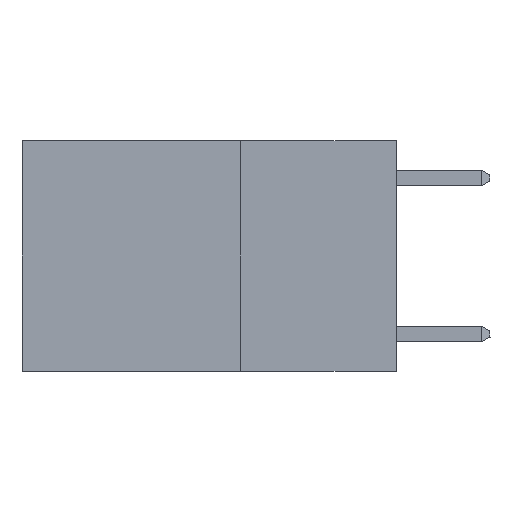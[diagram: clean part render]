
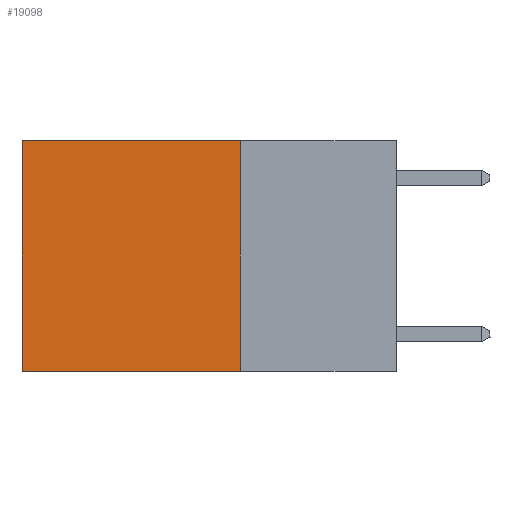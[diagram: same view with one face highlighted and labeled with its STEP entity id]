
A CAD part, left-side view. The second image highlights one B-rep face of the part: STEP entity #19098.
In plain terms, the highlighted planar face has unit normal (-1, 0, 0).
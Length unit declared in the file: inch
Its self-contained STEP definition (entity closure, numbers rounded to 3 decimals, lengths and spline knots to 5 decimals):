
#115 = CARTESIAN_POINT ( 'NONE',  ( 0.2625, 0.25, -0.37 ) ) ;
#633 = VECTOR ( 'NONE', #17100, 39.37008 ) ;
#937 = LINE ( 'NONE', #3452, #633 ) ;
#1127 = VERTEX_POINT ( 'NONE', #10724 ) ;
#1497 = EDGE_CURVE ( 'NONE', #13626, #9747, #11263, .T. ) ;
#1916 = DIRECTION ( 'NONE',  ( 0., 1., 0. ) ) ;
#2401 = PLANE ( 'NONE',  #7208 ) ;
#3452 = CARTESIAN_POINT ( 'NONE',  ( 0.2625, 0.25, 0. ) ) ;
#3915 = VECTOR ( 'NONE', #16270, 39.37008 ) ;
#4305 = ORIENTED_EDGE ( 'NONE', *, *, #17801, .F. ) ;
#5739 = ORIENTED_EDGE ( 'NONE', *, *, #16475, .T. ) ;
#6186 = DIRECTION ( 'NONE',  ( 0., 0., -1. ) ) ;
#6295 = CARTESIAN_POINT ( 'NONE',  ( 0.2625, 0.6, 0. ) ) ;
#7208 = AXIS2_PLACEMENT_3D ( 'NONE', #19495, #9434, #21037 ) ;
#7771 = CARTESIAN_POINT ( 'NONE',  ( 0.2625, 0.25, 0. ) ) ;
#8571 = LINE ( 'NONE', #7771, #3915 ) ;
#8834 = CARTESIAN_POINT ( 'NONE',  ( 0.2625, 0.6, -0.37 ) ) ;
#8914 = ORIENTED_EDGE ( 'NONE', *, *, #14545, .F. ) ;
#9434 = DIRECTION ( 'NONE',  ( 1., 0., 0. ) ) ;
#9747 = VERTEX_POINT ( 'NONE', #8834 ) ;
#10724 = CARTESIAN_POINT ( 'NONE',  ( 0.2625, 0.25, 0. ) ) ;
#10732 = VECTOR ( 'NONE', #6186, 39.37008 ) ;
#11263 = LINE ( 'NONE', #6295, #10732 ) ;
#12610 = ORIENTED_EDGE ( 'NONE', *, *, #1497, .T. ) ;
#13084 = FACE_OUTER_BOUND ( 'NONE', #19761, .T. ) ;
#13626 = VERTEX_POINT ( 'NONE', #19842 ) ;
#14545 = EDGE_CURVE ( 'NONE', #17948, #9747, #17337, .T. ) ;
#16270 = DIRECTION ( 'NONE',  ( 0., 0., -1. ) ) ;
#16475 = EDGE_CURVE ( 'NONE', #1127, #13626, #937, .T. ) ;
#17100 = DIRECTION ( 'NONE',  ( 0., 1., 0. ) ) ;
#17337 = LINE ( 'NONE', #115, #17551 ) ;
#17551 = VECTOR ( 'NONE', #1916, 39.37008 ) ;
#17801 = EDGE_CURVE ( 'NONE', #1127, #17948, #8571, .T. ) ;
#17948 = VERTEX_POINT ( 'NONE', #18332 ) ;
#18332 = CARTESIAN_POINT ( 'NONE',  ( 0.2625, 0.25, -0.37 ) ) ;
#19098 = ADVANCED_FACE ( 'NONE', ( #13084 ), #2401, .F. ) ;
#19495 = CARTESIAN_POINT ( 'NONE',  ( 0.2625, 0.25, 0. ) ) ;
#19761 = EDGE_LOOP ( 'NONE', ( #12610, #8914, #4305, #5739 ) ) ;
#19842 = CARTESIAN_POINT ( 'NONE',  ( 0.2625, 0.6, 0. ) ) ;
#21037 = DIRECTION ( 'NONE',  ( 0., 0., -1. ) ) ;
